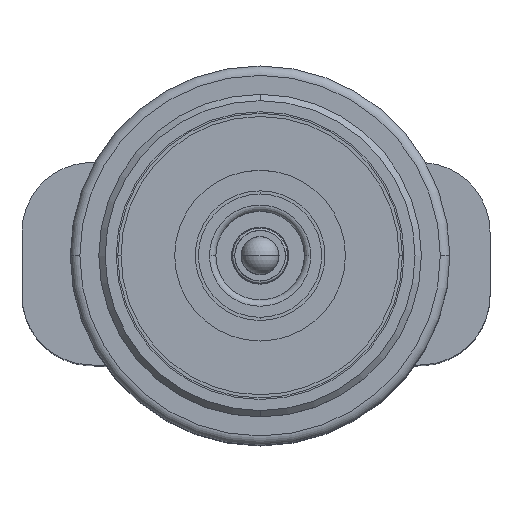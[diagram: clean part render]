
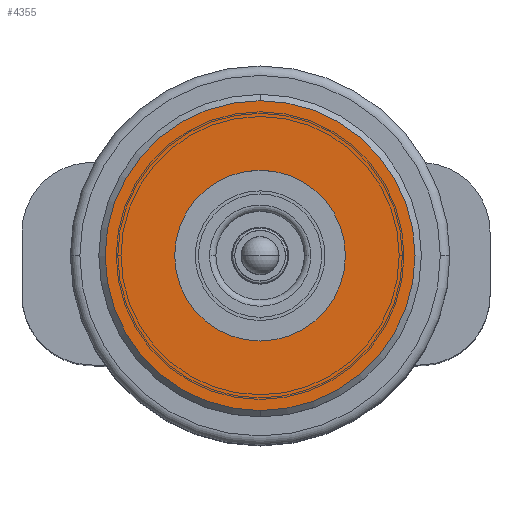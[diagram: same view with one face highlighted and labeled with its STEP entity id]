
A CAD part, top view. The second image highlights one B-rep face of the part: STEP entity #4355.
In plain terms, the highlighted planar face has unit normal (0, 0, 1).
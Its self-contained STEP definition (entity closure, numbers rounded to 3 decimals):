
#140 = ORIENTED_EDGE ( 'NONE', *, *, #567, .T. ) ;
#567 = EDGE_CURVE ( 'NONE', #5353, #5315, #3374, .T. ) ;
#656 = DIRECTION ( 'NONE',  ( 0., 0., 1. ) ) ;
#884 = CIRCLE ( 'NONE', #5818, 2.7 ) ;
#943 = EDGE_CURVE ( 'NONE', #6047, #3452, #884, .T. ) ;
#1082 = ORIENTED_EDGE ( 'NONE', *, *, #2123, .T. ) ;
#1212 = CARTESIAN_POINT ( 'NONE',  ( 20., 2.7, -5. ) ) ;
#1261 = CARTESIAN_POINT ( 'NONE',  ( 20., -4.9, -5. ) ) ;
#1321 = DIRECTION ( 'NONE',  ( 0., 0., 1. ) ) ;
#1330 = EDGE_LOOP ( 'NONE', ( #4910, #5846 ) ) ;
#1443 = CARTESIAN_POINT ( 'NONE',  ( 20., 0., -5. ) ) ;
#1499 = DIRECTION ( 'NONE',  ( 0., 0., 1. ) ) ;
#1712 = CIRCLE ( 'NONE', #5198, 4.9 ) ;
#2123 = EDGE_CURVE ( 'NONE', #5315, #5353, #1712, .T. ) ;
#2348 = CARTESIAN_POINT ( 'NONE',  ( 20., 0., -5. ) ) ;
#2462 = EDGE_CURVE ( 'NONE', #6047, #3452, #3990, .T. ) ;
#2798 = AXIS2_PLACEMENT_3D ( 'NONE', #5964, #656, #5046 ) ;
#2848 = CARTESIAN_POINT ( 'NONE',  ( 20., -2.7, -5. ) ) ;
#2929 = DIRECTION ( 'NONE',  ( 1., 0., 0. ) ) ;
#3266 = AXIS2_PLACEMENT_3D ( 'NONE', #5008, #3542, #3471 ) ;
#3374 = CIRCLE ( 'NONE', #2798, 4.9 ) ;
#3452 = VERTEX_POINT ( 'NONE', #2848 ) ;
#3460 = DIRECTION ( 'NONE',  ( 0., 1., 0. ) ) ;
#3471 = DIRECTION ( 'NONE',  ( 0., 1., 0. ) ) ;
#3542 = DIRECTION ( 'NONE',  ( 0., 0., 1. ) ) ;
#3744 = CARTESIAN_POINT ( 'NONE',  ( 20., 0., -5. ) ) ;
#3794 = EDGE_LOOP ( 'NONE', ( #1082, #140 ) ) ;
#3813 = CARTESIAN_POINT ( 'NONE',  ( 20., 4.9, -5. ) ) ;
#3892 = FACE_OUTER_BOUND ( 'NONE', #3794, .T. ) ;
#3990 = CIRCLE ( 'NONE', #3266, 2.7 ) ;
#4012 = DIRECTION ( 'NONE',  ( 0., 0., -1. ) ) ;
#4190 = DIRECTION ( 'NONE',  ( 0., 1., 0. ) ) ;
#4355 = ADVANCED_FACE ( 'NONE', ( #3892, #4468 ), #5849, .T. ) ;
#4468 = FACE_BOUND ( 'NONE', #1330, .T. ) ;
#4910 = ORIENTED_EDGE ( 'NONE', *, *, #2462, .F. ) ;
#5008 = CARTESIAN_POINT ( 'NONE',  ( 20., 0., -5. ) ) ;
#5046 = DIRECTION ( 'NONE',  ( 0., -1., 0. ) ) ;
#5198 = AXIS2_PLACEMENT_3D ( 'NONE', #3744, #1321, #4190 ) ;
#5315 = VERTEX_POINT ( 'NONE', #3813 ) ;
#5353 = VERTEX_POINT ( 'NONE', #1261 ) ;
#5818 = AXIS2_PLACEMENT_3D ( 'NONE', #2348, #4012, #3460 ) ;
#5846 = ORIENTED_EDGE ( 'NONE', *, *, #943, .T. ) ;
#5849 = PLANE ( 'NONE',  #6134 ) ;
#5964 = CARTESIAN_POINT ( 'NONE',  ( 20., 0., -5. ) ) ;
#6047 = VERTEX_POINT ( 'NONE', #1212 ) ;
#6134 = AXIS2_PLACEMENT_3D ( 'NONE', #1443, #1499, #2929 ) ;
